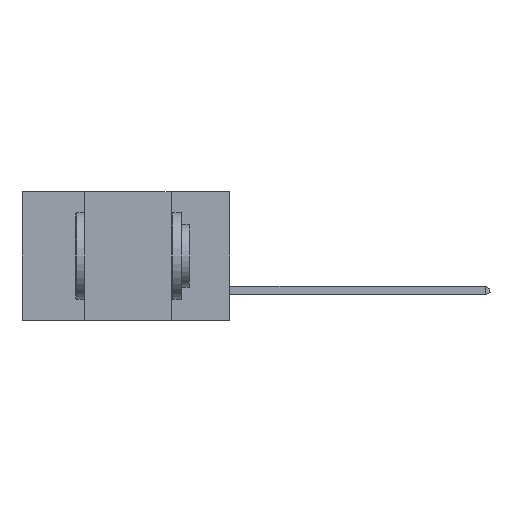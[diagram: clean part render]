
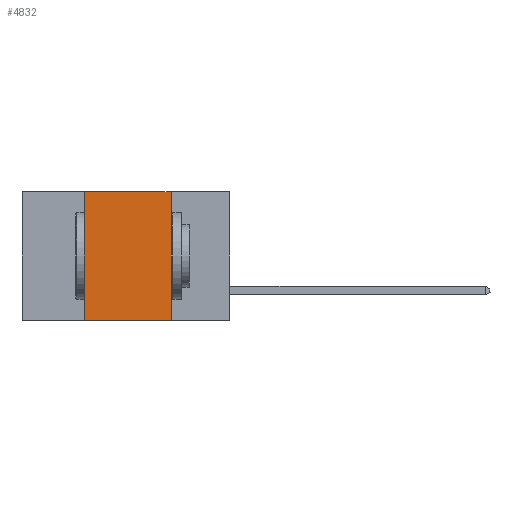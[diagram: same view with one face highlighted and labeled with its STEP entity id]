
A CAD part, left-side view. The second image highlights one B-rep face of the part: STEP entity #4832.
In plain terms, the highlighted planar face has unit normal (-1, 0, 0).
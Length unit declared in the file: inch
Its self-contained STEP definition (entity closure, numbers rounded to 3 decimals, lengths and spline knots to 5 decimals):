
#371 = DIRECTION ( 'NONE',  ( 0., 0., -1. ) ) ;
#1399 = CARTESIAN_POINT ( 'NONE',  ( 0., 0.17, 0. ) ) ;
#2459 = CARTESIAN_POINT ( 'NONE',  ( 0., 0.17, 0. ) ) ;
#2884 = VERTEX_POINT ( 'NONE', #10573 ) ;
#4459 = AXIS2_PLACEMENT_3D ( 'NONE', #17174, #29460, #7685 ) ;
#4832 = ADVANCED_FACE ( 'NONE', ( #25555 ), #29895, .F. ) ;
#5321 = CARTESIAN_POINT ( 'NONE',  ( 0., 0.6, 0. ) ) ;
#6164 = LINE ( 'NONE', #10591, #32025 ) ;
#6633 = ORIENTED_EDGE ( 'NONE', *, *, #12105, .F. ) ;
#7685 = DIRECTION ( 'NONE',  ( 0., 0., -1. ) ) ;
#9055 = VECTOR ( 'NONE', #17943, 39.37008 ) ;
#9748 = VECTOR ( 'NONE', #371, 39.37008 ) ;
#10573 = CARTESIAN_POINT ( 'NONE',  ( 0., 0.42, -0.37 ) ) ;
#10591 = CARTESIAN_POINT ( 'NONE',  ( 0., 0.6, -0.37 ) ) ;
#10807 = DIRECTION ( 'NONE',  ( 0., -1., 0. ) ) ;
#11286 = VERTEX_POINT ( 'NONE', #1399 ) ;
#12105 = EDGE_CURVE ( 'NONE', #22577, #11286, #22407, .T. ) ;
#12604 = EDGE_CURVE ( 'NONE', #2884, #22577, #22759, .T. ) ;
#12619 = ORIENTED_EDGE ( 'NONE', *, *, #21450, .T. ) ;
#14324 = DIRECTION ( 'NONE',  ( 0., 0., 1. ) ) ;
#17071 = EDGE_LOOP ( 'NONE', ( #17513, #6633, #19419, #12619 ) ) ;
#17174 = CARTESIAN_POINT ( 'NONE',  ( 0., 0.6, 0. ) ) ;
#17513 = ORIENTED_EDGE ( 'NONE', *, *, #28434, .F. ) ;
#17943 = DIRECTION ( 'NONE',  ( 0., -1., 0. ) ) ;
#19419 = ORIENTED_EDGE ( 'NONE', *, *, #12604, .F. ) ;
#21450 = EDGE_CURVE ( 'NONE', #2884, #24465, #6164, .T. ) ;
#22407 = LINE ( 'NONE', #5321, #9055 ) ;
#22577 = VERTEX_POINT ( 'NONE', #24194 ) ;
#22759 = LINE ( 'NONE', #26906, #30611 ) ;
#24134 = CARTESIAN_POINT ( 'NONE',  ( 0., 0.17, -0.37 ) ) ;
#24194 = CARTESIAN_POINT ( 'NONE',  ( 0., 0.42, 0. ) ) ;
#24465 = VERTEX_POINT ( 'NONE', #24134 ) ;
#25555 = FACE_OUTER_BOUND ( 'NONE', #17071, .T. ) ;
#26906 = CARTESIAN_POINT ( 'NONE',  ( 0., 0.42, 0. ) ) ;
#28434 = EDGE_CURVE ( 'NONE', #11286, #24465, #31730, .T. ) ;
#29460 = DIRECTION ( 'NONE',  ( 1., 0., 0. ) ) ;
#29895 = PLANE ( 'NONE',  #4459 ) ;
#30611 = VECTOR ( 'NONE', #14324, 39.37008 ) ;
#31730 = LINE ( 'NONE', #2459, #9748 ) ;
#32025 = VECTOR ( 'NONE', #10807, 39.37008 ) ;
